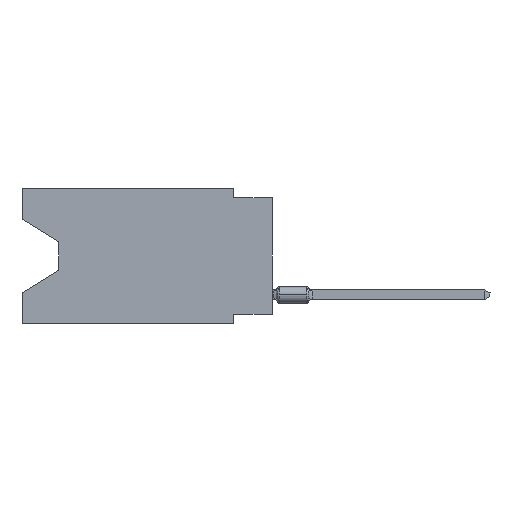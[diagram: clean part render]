
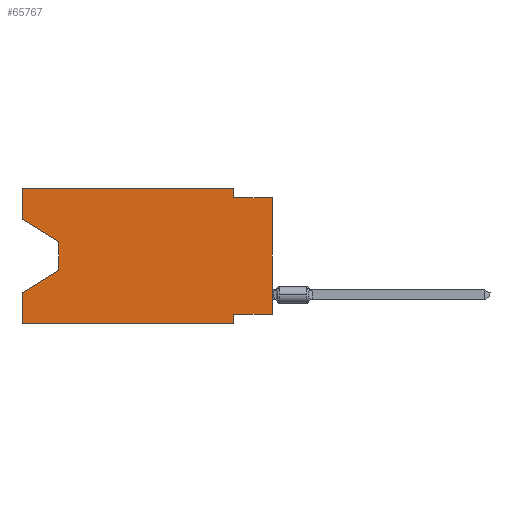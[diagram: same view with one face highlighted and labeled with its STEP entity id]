
A CAD part, left-side view. The second image highlights one B-rep face of the part: STEP entity #65767.
In plain terms, the highlighted planar face has unit normal (-1, 0, 0).
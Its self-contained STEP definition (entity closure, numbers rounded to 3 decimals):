
#1347 = CARTESIAN_POINT ( 'NONE',  ( 0., 16.383, -2.038 ) ) ;
#1735 = LINE ( 'NONE', #31656, #42535 ) ;
#2010 = LINE ( 'NONE', #50133, #55577 ) ;
#4528 = VERTEX_POINT ( 'NONE', #19934 ) ;
#6919 = ORIENTED_EDGE ( 'NONE', *, *, #8660, .F. ) ;
#8348 = CARTESIAN_POINT ( 'NONE',  ( 0., 16.383, -2.038 ) ) ;
#8648 = VECTOR ( 'NONE', #68241, 1000. ) ;
#8660 = EDGE_CURVE ( 'NONE', #36193, #75283, #58240, .T. ) ;
#8989 = VECTOR ( 'NONE', #43176, 1000. ) ;
#11079 = LINE ( 'NONE', #60821, #68476 ) ;
#11199 = AXIS2_PLACEMENT_3D ( 'NONE', #16333, #40988, #65665 ) ;
#11650 = VECTOR ( 'NONE', #24694, 1000. ) ;
#11761 = CARTESIAN_POINT ( 'NONE',  ( 0., 13.97, -3.505 ) ) ;
#13034 = ORIENTED_EDGE ( 'NONE', *, *, #61143, .F. ) ;
#13266 = LINE ( 'NONE', #19311, #8989 ) ;
#14693 = CARTESIAN_POINT ( 'NONE',  ( 0., 2.54, 0. ) ) ;
#16333 = CARTESIAN_POINT ( 'NONE',  ( 0., 16.383, 0. ) ) ;
#16646 = DIRECTION ( 'NONE',  ( 0., -1., 0. ) ) ;
#18512 = CARTESIAN_POINT ( 'NONE',  ( 0., 16.383, 0. ) ) ;
#19311 = CARTESIAN_POINT ( 'NONE',  ( 0., 16.383, 0. ) ) ;
#19373 = VECTOR ( 'NONE', #27516, 1000. ) ;
#19934 = CARTESIAN_POINT ( 'NONE',  ( 0., 0., -8.255 ) ) ;
#20367 = DIRECTION ( 'NONE',  ( 0., 0., 1. ) ) ;
#20613 = DIRECTION ( 'NONE',  ( 0., 0., 1. ) ) ;
#21017 = EDGE_CURVE ( 'NONE', #35292, #75283, #11079, .T. ) ;
#21215 = EDGE_CURVE ( 'NONE', #56515, #41744, #1735, .T. ) ;
#23659 = VERTEX_POINT ( 'NONE', #18512 ) ;
#23858 = ORIENTED_EDGE ( 'NONE', *, *, #41476, .T. ) ;
#24254 = VECTOR ( 'NONE', #44993, 1000. ) ;
#24694 = DIRECTION ( 'NONE',  ( 0., 0., -1. ) ) ;
#25445 = CARTESIAN_POINT ( 'NONE',  ( 0., 2.54, -8.89 ) ) ;
#25699 = ORIENTED_EDGE ( 'NONE', *, *, #40919, .T. ) ;
#26417 = LINE ( 'NONE', #1347, #24254 ) ;
#27516 = DIRECTION ( 'NONE',  ( 0., 0., -1. ) ) ;
#29833 = VECTOR ( 'NONE', #20367, 1000. ) ;
#30447 = CARTESIAN_POINT ( 'NONE',  ( 0., 0., -0.635 ) ) ;
#30633 = LINE ( 'NONE', #67448, #8648 ) ;
#30891 = CARTESIAN_POINT ( 'NONE',  ( 0., 16.383, -6.852 ) ) ;
#31656 = CARTESIAN_POINT ( 'NONE',  ( 0., 0., -0.635 ) ) ;
#31668 = EDGE_CURVE ( 'NONE', #35659, #56515, #48370, .T. ) ;
#32360 = CARTESIAN_POINT ( 'NONE',  ( 0., 13.97, -5.385 ) ) ;
#32937 = CARTESIAN_POINT ( 'NONE',  ( 0., 13.97, -5.385 ) ) ;
#33335 = EDGE_CURVE ( 'NONE', #43227, #51896, #26417, .T. ) ;
#35292 = VERTEX_POINT ( 'NONE', #43992 ) ;
#35659 = VERTEX_POINT ( 'NONE', #14693 ) ;
#36193 = VERTEX_POINT ( 'NONE', #45728 ) ;
#37781 = LINE ( 'NONE', #62457, #29833 ) ;
#38828 = EDGE_LOOP ( 'NONE', ( #63717, #25699, #23858, #39842, #61660, #6919, #62699, #42047, #45467, #65791, #13034, #77142 ) ) ;
#38929 = DIRECTION ( 'NONE',  ( 0., -1., 0. ) ) ;
#39842 = ORIENTED_EDGE ( 'NONE', *, *, #63199, .F. ) ;
#40019 = CARTESIAN_POINT ( 'NONE',  ( 0., 2.54, -8.89 ) ) ;
#40919 = EDGE_CURVE ( 'NONE', #51896, #54968, #61105, .T. ) ;
#40988 = DIRECTION ( 'NONE',  ( 1., 0., 0. ) ) ;
#41104 = EDGE_CURVE ( 'NONE', #4528, #41744, #2010, .T. ) ;
#41476 = EDGE_CURVE ( 'NONE', #54968, #54597, #58423, .T. ) ;
#41744 = VERTEX_POINT ( 'NONE', #30447 ) ;
#42047 = ORIENTED_EDGE ( 'NONE', *, *, #41104, .T. ) ;
#42535 = VECTOR ( 'NONE', #38929, 1000. ) ;
#43176 = DIRECTION ( 'NONE',  ( 0., 0., 1. ) ) ;
#43227 = VERTEX_POINT ( 'NONE', #8348 ) ;
#43992 = CARTESIAN_POINT ( 'NONE',  ( 0., 16.383, -8.89 ) ) ;
#44993 = DIRECTION ( 'NONE',  ( 0., -0.855, -0.519 ) ) ;
#45467 = ORIENTED_EDGE ( 'NONE', *, *, #21215, .F. ) ;
#45728 = CARTESIAN_POINT ( 'NONE',  ( 0., 2.54, -8.255 ) ) ;
#45872 = LINE ( 'NONE', #51944, #73487 ) ;
#46580 = VECTOR ( 'NONE', #52730, 1000. ) ;
#47947 = CARTESIAN_POINT ( 'NONE',  ( 0., 2.54, -0.635 ) ) ;
#48370 = LINE ( 'NONE', #67766, #55078 ) ;
#50133 = CARTESIAN_POINT ( 'NONE',  ( 0., 0., 0. ) ) ;
#51896 = VERTEX_POINT ( 'NONE', #52662 ) ;
#51944 = CARTESIAN_POINT ( 'NONE',  ( 0., 16.383, 0. ) ) ;
#52662 = CARTESIAN_POINT ( 'NONE',  ( 0., 13.97, -3.505 ) ) ;
#52730 = DIRECTION ( 'NONE',  ( 0., 0.855, -0.519 ) ) ;
#53127 = PLANE ( 'NONE',  #11199 ) ;
#54597 = VERTEX_POINT ( 'NONE', #30891 ) ;
#54968 = VERTEX_POINT ( 'NONE', #32360 ) ;
#55078 = VECTOR ( 'NONE', #79122, 1000. ) ;
#55577 = VECTOR ( 'NONE', #20613, 1000. ) ;
#56515 = VERTEX_POINT ( 'NONE', #47947 ) ;
#58240 = LINE ( 'NONE', #40019, #19373 ) ;
#58423 = LINE ( 'NONE', #32937, #46580 ) ;
#59206 = FACE_OUTER_BOUND ( 'NONE', #38828, .T. ) ;
#60821 = CARTESIAN_POINT ( 'NONE',  ( 0., 16.383, -8.89 ) ) ;
#61105 = LINE ( 'NONE', #11761, #11650 ) ;
#61143 = EDGE_CURVE ( 'NONE', #23659, #35659, #45872, .T. ) ;
#61660 = ORIENTED_EDGE ( 'NONE', *, *, #21017, .T. ) ;
#61775 = EDGE_CURVE ( 'NONE', #43227, #23659, #13266, .T. ) ;
#62457 = CARTESIAN_POINT ( 'NONE',  ( 0., 16.383, 0. ) ) ;
#62699 = ORIENTED_EDGE ( 'NONE', *, *, #65623, .F. ) ;
#63199 = EDGE_CURVE ( 'NONE', #35292, #54597, #37781, .T. ) ;
#63717 = ORIENTED_EDGE ( 'NONE', *, *, #33335, .T. ) ;
#65623 = EDGE_CURVE ( 'NONE', #4528, #36193, #30633, .T. ) ;
#65665 = DIRECTION ( 'NONE',  ( 0., 0., -1. ) ) ;
#65767 = ADVANCED_FACE ( 'NONE', ( #59206 ), #53127, .F. ) ;
#65791 = ORIENTED_EDGE ( 'NONE', *, *, #31668, .F. ) ;
#67448 = CARTESIAN_POINT ( 'NONE',  ( 0., 0., -8.255 ) ) ;
#67766 = CARTESIAN_POINT ( 'NONE',  ( 0., 2.54, 0. ) ) ;
#68241 = DIRECTION ( 'NONE',  ( 0., 1., 0. ) ) ;
#68476 = VECTOR ( 'NONE', #73753, 1000. ) ;
#73487 = VECTOR ( 'NONE', #16646, 1000. ) ;
#73753 = DIRECTION ( 'NONE',  ( 0., -1., 0. ) ) ;
#75283 = VERTEX_POINT ( 'NONE', #25445 ) ;
#77142 = ORIENTED_EDGE ( 'NONE', *, *, #61775, .F. ) ;
#79122 = DIRECTION ( 'NONE',  ( 0., 0., -1. ) ) ;
